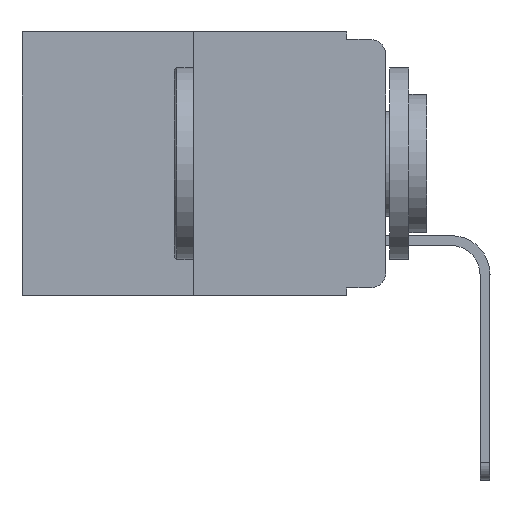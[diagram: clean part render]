
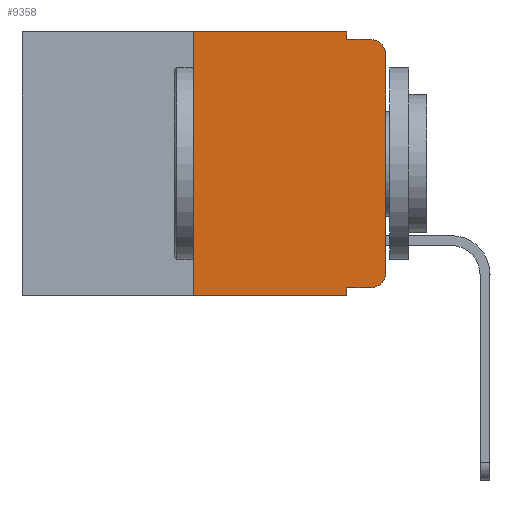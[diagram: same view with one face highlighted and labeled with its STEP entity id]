
A CAD part, left-side view. The second image highlights one B-rep face of the part: STEP entity #9358.
In plain terms, the highlighted planar face has unit normal (-1, 0, 0).
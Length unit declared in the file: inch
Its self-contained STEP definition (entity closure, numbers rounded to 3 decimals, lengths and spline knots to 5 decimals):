
#271 = LINE ( 'NONE', #3932, #11154 ) ;
#371 = CARTESIAN_POINT ( 'NONE',  ( 0., 0.02, -0.313 ) ) ;
#611 = LINE ( 'NONE', #6903, #12824 ) ;
#811 = AXIS2_PLACEMENT_3D ( 'NONE', #5458, #3295, #7678 ) ;
#958 = VECTOR ( 'NONE', #11856, 39.37008 ) ;
#1024 = CARTESIAN_POINT ( 'NONE',  ( 0., 0.25, 0. ) ) ;
#1311 = CARTESIAN_POINT ( 'NONE',  ( 0., 0.051, -0.01 ) ) ;
#1472 = VECTOR ( 'NONE', #5738, 39.37008 ) ;
#1568 = VERTEX_POINT ( 'NONE', #2030 ) ;
#1608 = VERTEX_POINT ( 'NONE', #5370 ) ;
#1871 = CARTESIAN_POINT ( 'NONE',  ( 0., 0.051, -0.343 ) ) ;
#2030 = CARTESIAN_POINT ( 'NONE',  ( 0., 0.02, -0.01 ) ) ;
#2342 = CARTESIAN_POINT ( 'NONE',  ( 0., 0.25, -0.343 ) ) ;
#2691 = ORIENTED_EDGE ( 'NONE', *, *, #5926, .T. ) ;
#2845 = ORIENTED_EDGE ( 'NONE', *, *, #4747, .T. ) ;
#2850 = AXIS2_PLACEMENT_3D ( 'NONE', #371, #6727, #7879 ) ;
#2934 = DIRECTION ( 'NONE',  ( 0., -1., 0. ) ) ;
#3002 = VERTEX_POINT ( 'NONE', #12957 ) ;
#3085 = ORIENTED_EDGE ( 'NONE', *, *, #9393, .F. ) ;
#3295 = DIRECTION ( 'NONE',  ( -1., 0., 0. ) ) ;
#3331 = CARTESIAN_POINT ( 'NONE',  ( 0., 0., 0. ) ) ;
#3373 = DIRECTION ( 'NONE',  ( 0., 0., 1. ) ) ;
#3408 = ORIENTED_EDGE ( 'NONE', *, *, #8901, .T. ) ;
#3772 = ORIENTED_EDGE ( 'NONE', *, *, #10116, .F. ) ;
#3861 = VERTEX_POINT ( 'NONE', #12691 ) ;
#3932 = CARTESIAN_POINT ( 'NONE',  ( 0., 0.473, 0. ) ) ;
#4055 = LINE ( 'NONE', #3331, #9017 ) ;
#4533 = ORIENTED_EDGE ( 'NONE', *, *, #6007, .F. ) ;
#4581 = LINE ( 'NONE', #13131, #1472 ) ;
#4679 = VECTOR ( 'NONE', #11328, 39.37008 ) ;
#4747 = EDGE_CURVE ( 'NONE', #10218, #6974, #6036, .T. ) ;
#5064 = DIRECTION ( 'NONE',  ( 0., -1., 0. ) ) ;
#5364 = PLANE ( 'NONE',  #11069 ) ;
#5370 = CARTESIAN_POINT ( 'NONE',  ( 0., 0.051, 0. ) ) ;
#5458 = CARTESIAN_POINT ( 'NONE',  ( 0., 0.02, -0.03 ) ) ;
#5634 = EDGE_CURVE ( 'NONE', #3002, #1568, #8698, .T. ) ;
#5714 = VECTOR ( 'NONE', #5064, 39.37008 ) ;
#5738 = DIRECTION ( 'NONE',  ( 0., 0., 1. ) ) ;
#5926 = EDGE_CURVE ( 'NONE', #6954, #10137, #611, .T. ) ;
#6007 = EDGE_CURVE ( 'NONE', #9273, #1608, #271, .T. ) ;
#6019 = CARTESIAN_POINT ( 'NONE',  ( 0., 0.051, -0.333 ) ) ;
#6036 = LINE ( 'NONE', #6019, #5714 ) ;
#6209 = LINE ( 'NONE', #1311, #12669 ) ;
#6262 = EDGE_CURVE ( 'NONE', #3861, #3002, #4055, .T. ) ;
#6263 = ORIENTED_EDGE ( 'NONE', *, *, #5634, .T. ) ;
#6619 = ORIENTED_EDGE ( 'NONE', *, *, #12114, .F. ) ;
#6727 = DIRECTION ( 'NONE',  ( -1., 0., 0. ) ) ;
#6820 = EDGE_LOOP ( 'NONE', ( #7742, #6263, #3772, #3085, #4533, #8410, #2691, #6619, #2845, #3408 ) ) ;
#6903 = CARTESIAN_POINT ( 'NONE',  ( 0., 0.473, -0.343 ) ) ;
#6954 = VERTEX_POINT ( 'NONE', #2342 ) ;
#6974 = VERTEX_POINT ( 'NONE', #7603 ) ;
#7289 = CIRCLE ( 'NONE', #2850, 0.02 ) ;
#7492 = LINE ( 'NONE', #9165, #4679 ) ;
#7603 = CARTESIAN_POINT ( 'NONE',  ( 0., 0.02, -0.333 ) ) ;
#7618 = CARTESIAN_POINT ( 'NONE',  ( 0., 0.051, -0.01 ) ) ;
#7678 = DIRECTION ( 'NONE',  ( 0., 0., -1. ) ) ;
#7742 = ORIENTED_EDGE ( 'NONE', *, *, #6262, .T. ) ;
#7816 = FACE_OUTER_BOUND ( 'NONE', #6820, .T. ) ;
#7879 = DIRECTION ( 'NONE',  ( 0., 0., -1. ) ) ;
#8041 = DIRECTION ( 'NONE',  ( 0., -1., 0. ) ) ;
#8410 = ORIENTED_EDGE ( 'NONE', *, *, #9522, .F. ) ;
#8698 = CIRCLE ( 'NONE', #811, 0.02 ) ;
#8901 = EDGE_CURVE ( 'NONE', #6974, #3861, #7289, .T. ) ;
#9017 = VECTOR ( 'NONE', #3373, 39.37008 ) ;
#9056 = LINE ( 'NONE', #10731, #958 ) ;
#9165 = CARTESIAN_POINT ( 'NONE',  ( 0., 0.051, 0. ) ) ;
#9273 = VERTEX_POINT ( 'NONE', #1024 ) ;
#9358 = ADVANCED_FACE ( 'NONE', ( #7816 ), #5364, .F. ) ;
#9393 = EDGE_CURVE ( 'NONE', #1608, #10741, #9056, .T. ) ;
#9486 = CARTESIAN_POINT ( 'NONE',  ( 0., 0.473, 0. ) ) ;
#9522 = EDGE_CURVE ( 'NONE', #6954, #9273, #4581, .T. ) ;
#10108 = DIRECTION ( 'NONE',  ( 0., -1., 0. ) ) ;
#10116 = EDGE_CURVE ( 'NONE', #10741, #1568, #6209, .T. ) ;
#10137 = VERTEX_POINT ( 'NONE', #1871 ) ;
#10218 = VERTEX_POINT ( 'NONE', #10343 ) ;
#10343 = CARTESIAN_POINT ( 'NONE',  ( 0., 0.051, -0.333 ) ) ;
#10731 = CARTESIAN_POINT ( 'NONE',  ( 0., 0.051, 0. ) ) ;
#10741 = VERTEX_POINT ( 'NONE', #7618 ) ;
#11069 = AXIS2_PLACEMENT_3D ( 'NONE', #9486, #12955, #12819 ) ;
#11154 = VECTOR ( 'NONE', #2934, 39.37008 ) ;
#11328 = DIRECTION ( 'NONE',  ( 0., 0., -1. ) ) ;
#11856 = DIRECTION ( 'NONE',  ( 0., 0., -1. ) ) ;
#12114 = EDGE_CURVE ( 'NONE', #10218, #10137, #7492, .T. ) ;
#12669 = VECTOR ( 'NONE', #8041, 39.37008 ) ;
#12691 = CARTESIAN_POINT ( 'NONE',  ( 0., 0., -0.313 ) ) ;
#12819 = DIRECTION ( 'NONE',  ( 0., 0., -1. ) ) ;
#12824 = VECTOR ( 'NONE', #10108, 39.37008 ) ;
#12955 = DIRECTION ( 'NONE',  ( 1., 0., 0. ) ) ;
#12957 = CARTESIAN_POINT ( 'NONE',  ( 0., 0., -0.03 ) ) ;
#13131 = CARTESIAN_POINT ( 'NONE',  ( 0., 0.25, 0. ) ) ;
